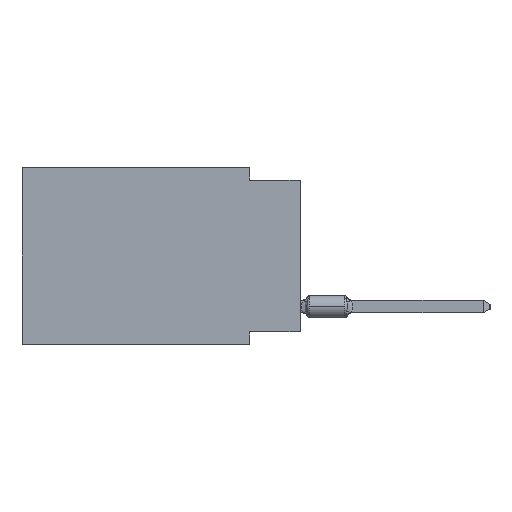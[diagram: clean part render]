
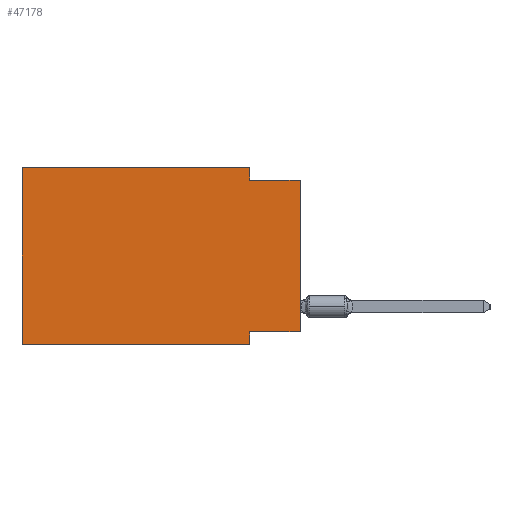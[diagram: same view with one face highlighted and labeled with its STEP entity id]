
A CAD part, left-side view. The second image highlights one B-rep face of the part: STEP entity #47178.
In plain terms, the highlighted planar face has unit normal (-1, 0, 0).
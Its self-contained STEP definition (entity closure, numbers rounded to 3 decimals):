
#2738 = EDGE_CURVE ( 'NONE', #56763, #45830, #27839, .T. ) ;
#5575 = VERTEX_POINT ( 'NONE', #18571 ) ;
#6265 = FACE_OUTER_BOUND ( 'NONE', #33853, .T. ) ;
#6603 = CARTESIAN_POINT ( 'NONE',  ( 0., 13.97, 0. ) ) ;
#6913 = ORIENTED_EDGE ( 'NONE', *, *, #62886, .F. ) ;
#7403 = VECTOR ( 'NONE', #36924, 1000. ) ;
#7853 = DIRECTION ( 'NONE',  ( 0., 0., 1. ) ) ;
#8815 = VECTOR ( 'NONE', #31978, 1000. ) ;
#9455 = AXIS2_PLACEMENT_3D ( 'NONE', #6603, #31979, #58007 ) ;
#10368 = CARTESIAN_POINT ( 'NONE',  ( 0., 13.97, 0. ) ) ;
#11588 = LINE ( 'NONE', #58519, #63130 ) ;
#14633 = DIRECTION ( 'NONE',  ( 0., -1., 0. ) ) ;
#14687 = ORIENTED_EDGE ( 'NONE', *, *, #48688, .F. ) ;
#14752 = CARTESIAN_POINT ( 'NONE',  ( 0., 2.54, -0.635 ) ) ;
#15671 = CARTESIAN_POINT ( 'NONE',  ( 0., 13.97, -8.89 ) ) ;
#17467 = EDGE_CURVE ( 'NONE', #24574, #62991, #67693, .T. ) ;
#18571 = CARTESIAN_POINT ( 'NONE',  ( 0., 0., -8.255 ) ) ;
#21351 = PLANE ( 'NONE',  #9455 ) ;
#22942 = DIRECTION ( 'NONE',  ( 0., 0., -1. ) ) ;
#23062 = ORIENTED_EDGE ( 'NONE', *, *, #2738, .F. ) ;
#24574 = VERTEX_POINT ( 'NONE', #40394 ) ;
#25857 = CARTESIAN_POINT ( 'NONE',  ( 0., 2.54, 0. ) ) ;
#26285 = LINE ( 'NONE', #15671, #7403 ) ;
#26682 = EDGE_CURVE ( 'NONE', #56763, #62991, #26285, .T. ) ;
#26819 = VECTOR ( 'NONE', #7853, 1000. ) ;
#27169 = CARTESIAN_POINT ( 'NONE',  ( 0., 13.97, 0. ) ) ;
#27347 = DIRECTION ( 'NONE',  ( 0., 1., 0. ) ) ;
#27839 = LINE ( 'NONE', #27169, #8815 ) ;
#29635 = VECTOR ( 'NONE', #62208, 1000. ) ;
#30126 = VECTOR ( 'NONE', #22942, 1000. ) ;
#30541 = CARTESIAN_POINT ( 'NONE',  ( 0., 13.97, 0. ) ) ;
#31978 = DIRECTION ( 'NONE',  ( 0., 0., 1. ) ) ;
#31979 = DIRECTION ( 'NONE',  ( 1., 0., 0. ) ) ;
#33320 = VERTEX_POINT ( 'NONE', #14752 ) ;
#33853 = EDGE_LOOP ( 'NONE', ( #64886, #6913, #53311, #14687, #23062, #39024, #42591, #42166 ) ) ;
#34874 = CARTESIAN_POINT ( 'NONE',  ( 0., 0., -0.635 ) ) ;
#36924 = DIRECTION ( 'NONE',  ( 0., -1., 0. ) ) ;
#37332 = VERTEX_POINT ( 'NONE', #62514 ) ;
#39024 = ORIENTED_EDGE ( 'NONE', *, *, #26682, .T. ) ;
#40394 = CARTESIAN_POINT ( 'NONE',  ( 0., 2.54, -8.255 ) ) ;
#41314 = VECTOR ( 'NONE', #51495, 1000. ) ;
#42166 = ORIENTED_EDGE ( 'NONE', *, *, #47638, .F. ) ;
#42591 = ORIENTED_EDGE ( 'NONE', *, *, #17467, .F. ) ;
#42830 = VERTEX_POINT ( 'NONE', #25857 ) ;
#44869 = CARTESIAN_POINT ( 'NONE',  ( 0., 0., 0. ) ) ;
#45830 = VERTEX_POINT ( 'NONE', #30541 ) ;
#45948 = EDGE_CURVE ( 'NONE', #42830, #33320, #58241, .T. ) ;
#46160 = EDGE_CURVE ( 'NONE', #5575, #37332, #54802, .T. ) ;
#47178 = ADVANCED_FACE ( 'NONE', ( #6265 ), #21351, .F. ) ;
#47638 = EDGE_CURVE ( 'NONE', #5575, #24574, #11588, .T. ) ;
#48688 = EDGE_CURVE ( 'NONE', #45830, #42830, #51824, .T. ) ;
#50561 = CARTESIAN_POINT ( 'NONE',  ( 0., 2.54, -8.89 ) ) ;
#51495 = DIRECTION ( 'NONE',  ( 0., -1., 0. ) ) ;
#51824 = LINE ( 'NONE', #10368, #41314 ) ;
#53101 = CARTESIAN_POINT ( 'NONE',  ( 0., 2.54, 0. ) ) ;
#53311 = ORIENTED_EDGE ( 'NONE', *, *, #45948, .F. ) ;
#54802 = LINE ( 'NONE', #44869, #26819 ) ;
#56763 = VERTEX_POINT ( 'NONE', #59896 ) ;
#58007 = DIRECTION ( 'NONE',  ( 0., 0., -1. ) ) ;
#58241 = LINE ( 'NONE', #53101, #30126 ) ;
#58519 = CARTESIAN_POINT ( 'NONE',  ( 0., 0., -8.255 ) ) ;
#59896 = CARTESIAN_POINT ( 'NONE',  ( 0., 13.97, -8.89 ) ) ;
#60242 = LINE ( 'NONE', #34874, #60851 ) ;
#60851 = VECTOR ( 'NONE', #14633, 1000. ) ;
#62208 = DIRECTION ( 'NONE',  ( 0., 0., -1. ) ) ;
#62514 = CARTESIAN_POINT ( 'NONE',  ( 0., 0., -0.635 ) ) ;
#62886 = EDGE_CURVE ( 'NONE', #33320, #37332, #60242, .T. ) ;
#62991 = VERTEX_POINT ( 'NONE', #65713 ) ;
#63130 = VECTOR ( 'NONE', #27347, 1000. ) ;
#64886 = ORIENTED_EDGE ( 'NONE', *, *, #46160, .T. ) ;
#65713 = CARTESIAN_POINT ( 'NONE',  ( 0., 2.54, -8.89 ) ) ;
#67693 = LINE ( 'NONE', #50561, #29635 ) ;
